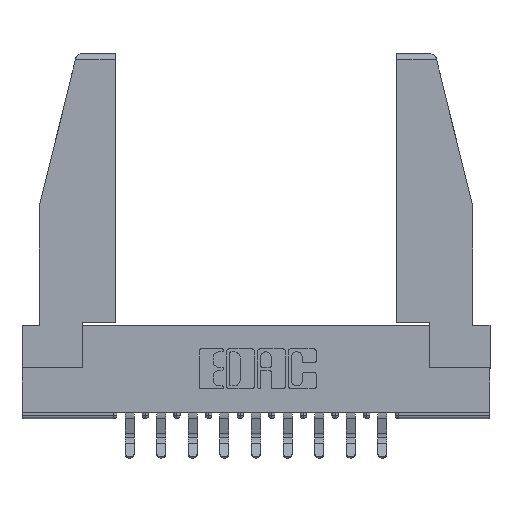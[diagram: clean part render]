
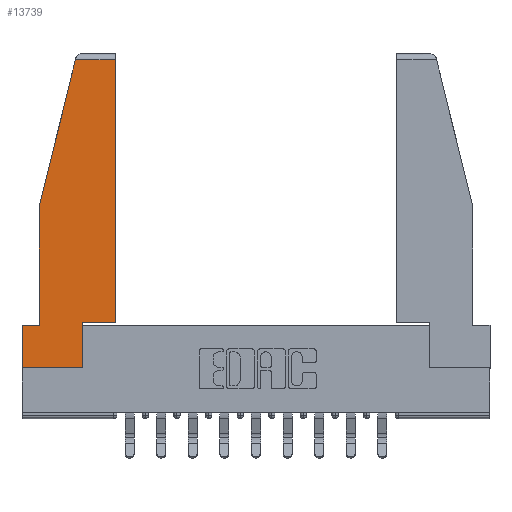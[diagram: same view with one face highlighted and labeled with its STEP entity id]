
A CAD part, top view. The second image highlights one B-rep face of the part: STEP entity #13739.
In plain terms, the highlighted planar face has unit normal (0, 0, 1).
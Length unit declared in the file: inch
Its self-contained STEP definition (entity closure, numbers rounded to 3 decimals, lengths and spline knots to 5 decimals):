
#1 = LINE ( 'NONE', #12663, #1201 ) ;
#361 = CARTESIAN_POINT ( 'NONE',  ( 0.086, 0.21, 0. ) ) ;
#486 = VECTOR ( 'NONE', #3379, 39.37008 ) ;
#639 = ORIENTED_EDGE ( 'NONE', *, *, #8112, .T. ) ;
#884 = LINE ( 'NONE', #13699, #486 ) ;
#1199 = EDGE_LOOP ( 'NONE', ( #13200, #10818, #13336, #12630, #14431, #3771, #639, #15785, #2026 ) ) ;
#1201 = VECTOR ( 'NONE', #16442, 39.37008 ) ;
#1258 = DIRECTION ( 'NONE',  ( -0.239, -0.971, 0. ) ) ;
#1736 = LINE ( 'NONE', #3740, #13220 ) ;
#1867 = LINE ( 'NONE', #15370, #16357 ) ;
#2005 = DIRECTION ( 'NONE',  ( 1., 0., 0. ) ) ;
#2026 = ORIENTED_EDGE ( 'NONE', *, *, #7312, .T. ) ;
#2544 = DIRECTION ( 'NONE',  ( 1., 0., 0. ) ) ;
#3379 = DIRECTION ( 'NONE',  ( 1., 0., 0. ) ) ;
#3740 = CARTESIAN_POINT ( 'NONE',  ( 0.271, 1.55, 0. ) ) ;
#3771 = ORIENTED_EDGE ( 'NONE', *, *, #7905, .T. ) ;
#4245 = VECTOR ( 'NONE', #10683, 39.37008 ) ;
#4628 = DIRECTION ( 'NONE',  ( 0., -1., 0. ) ) ;
#5558 = VERTEX_POINT ( 'NONE', #6913 ) ;
#6661 = EDGE_CURVE ( 'NONE', #10542, #13276, #1736, .T. ) ;
#6887 = VERTEX_POINT ( 'NONE', #361 ) ;
#6913 = CARTESIAN_POINT ( 'NONE',  ( 0.461, 0.223, 0. ) ) ;
#6998 = FACE_OUTER_BOUND ( 'NONE', #1199, .T. ) ;
#7025 = VERTEX_POINT ( 'NONE', #7537 ) ;
#7147 = CARTESIAN_POINT ( 'NONE',  ( 0., 1.52, 0. ) ) ;
#7245 = VECTOR ( 'NONE', #12987, 39.37008 ) ;
#7312 = EDGE_CURVE ( 'NONE', #13316, #5558, #9205, .T. ) ;
#7454 = VECTOR ( 'NONE', #2005, 39.37008 ) ;
#7537 = CARTESIAN_POINT ( 'NONE',  ( 0., 0., 0. ) ) ;
#7594 = PLANE ( 'NONE',  #8521 ) ;
#7765 = VECTOR ( 'NONE', #16065, 39.37008 ) ;
#7849 = EDGE_CURVE ( 'NONE', #6887, #10429, #12403, .T. ) ;
#7905 = EDGE_CURVE ( 'NONE', #10429, #7025, #15363, .T. ) ;
#8112 = EDGE_CURVE ( 'NONE', #7025, #9026, #884, .T. ) ;
#8338 = CARTESIAN_POINT ( 'NONE',  ( 0.297, 0., 0. ) ) ;
#8521 = AXIS2_PLACEMENT_3D ( 'NONE', #16370, #10112, #2544 ) ;
#8522 = LINE ( 'NONE', #12396, #12514 ) ;
#8561 = VERTEX_POINT ( 'NONE', #14604 ) ;
#9026 = VERTEX_POINT ( 'NONE', #8338 ) ;
#9205 = LINE ( 'NONE', #10730, #7454 ) ;
#10112 = DIRECTION ( 'NONE',  ( 0., 0., 1. ) ) ;
#10429 = VERTEX_POINT ( 'NONE', #14024 ) ;
#10542 = VERTEX_POINT ( 'NONE', #13529 ) ;
#10683 = DIRECTION ( 'NONE',  ( 0., -1., 0. ) ) ;
#10730 = CARTESIAN_POINT ( 'NONE',  ( 0.297, 0.223, 0. ) ) ;
#10818 = ORIENTED_EDGE ( 'NONE', *, *, #14089, .T. ) ;
#11810 = CARTESIAN_POINT ( 'NONE',  ( 0., 0.21, 0. ) ) ;
#12125 = LINE ( 'NONE', #7147, #7765 ) ;
#12396 = CARTESIAN_POINT ( 'NONE',  ( 0.086, 0.8, 0. ) ) ;
#12403 = LINE ( 'NONE', #11810, #7245 ) ;
#12514 = VECTOR ( 'NONE', #4628, 39.37008 ) ;
#12630 = ORIENTED_EDGE ( 'NONE', *, *, #14377, .T. ) ;
#12663 = CARTESIAN_POINT ( 'NONE',  ( 0.461, 0.223, 0. ) ) ;
#12765 = CARTESIAN_POINT ( 'NONE',  ( 0.297, 0.223, 0. ) ) ;
#12854 = EDGE_CURVE ( 'NONE', #9026, #13316, #1867, .T. ) ;
#12929 = CARTESIAN_POINT ( 'NONE',  ( 0.086, 0.8, 0. ) ) ;
#12987 = DIRECTION ( 'NONE',  ( -1., 0., 0. ) ) ;
#13200 = ORIENTED_EDGE ( 'NONE', *, *, #14712, .T. ) ;
#13220 = VECTOR ( 'NONE', #1258, 39.37008 ) ;
#13276 = VERTEX_POINT ( 'NONE', #12929 ) ;
#13316 = VERTEX_POINT ( 'NONE', #12765 ) ;
#13336 = ORIENTED_EDGE ( 'NONE', *, *, #6661, .T. ) ;
#13529 = CARTESIAN_POINT ( 'NONE',  ( 0.2636, 1.52, 0. ) ) ;
#13699 = CARTESIAN_POINT ( 'NONE',  ( 0., 0., 0. ) ) ;
#13739 = ADVANCED_FACE ( 'NONE', ( #6998 ), #7594, .T. ) ;
#14024 = CARTESIAN_POINT ( 'NONE',  ( 0., 0.21, 0. ) ) ;
#14089 = EDGE_CURVE ( 'NONE', #8561, #10542, #12125, .T. ) ;
#14261 = DIRECTION ( 'NONE',  ( 0., 1., 0. ) ) ;
#14377 = EDGE_CURVE ( 'NONE', #13276, #6887, #8522, .T. ) ;
#14431 = ORIENTED_EDGE ( 'NONE', *, *, #7849, .T. ) ;
#14604 = CARTESIAN_POINT ( 'NONE',  ( 0.461, 1.52, 0. ) ) ;
#14704 = CARTESIAN_POINT ( 'NONE',  ( 0., 0.21, 0. ) ) ;
#14712 = EDGE_CURVE ( 'NONE', #5558, #8561, #1, .T. ) ;
#15363 = LINE ( 'NONE', #14704, #4245 ) ;
#15370 = CARTESIAN_POINT ( 'NONE',  ( 0.297, 0., 0. ) ) ;
#15785 = ORIENTED_EDGE ( 'NONE', *, *, #12854, .T. ) ;
#16065 = DIRECTION ( 'NONE',  ( -1., 0., 0. ) ) ;
#16357 = VECTOR ( 'NONE', #14261, 39.37008 ) ;
#16370 = CARTESIAN_POINT ( 'NONE',  ( 0., 0., 0. ) ) ;
#16442 = DIRECTION ( 'NONE',  ( 0., 1., 0. ) ) ;
